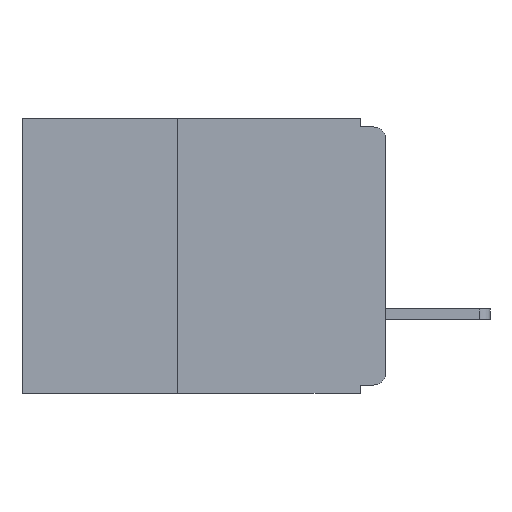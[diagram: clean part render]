
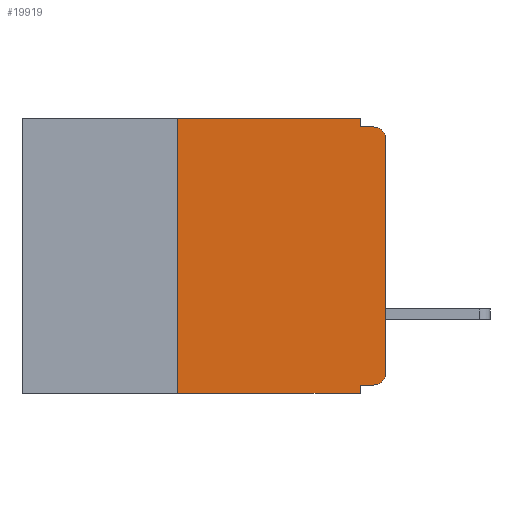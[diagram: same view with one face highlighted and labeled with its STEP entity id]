
A CAD part, left-side view. The second image highlights one B-rep face of the part: STEP entity #19919.
In plain terms, the highlighted planar face has unit normal (-1, 0, 0).
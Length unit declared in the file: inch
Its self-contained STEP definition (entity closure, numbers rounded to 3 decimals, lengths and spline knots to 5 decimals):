
#400 = LINE ( 'NONE', #5415, #15507 ) ;
#1231 = CARTESIAN_POINT ( 'NONE',  ( 0., 0., -0.305 ) ) ;
#1359 = EDGE_CURVE ( 'NONE', #19002, #3537, #1965, .T. ) ;
#1644 = CARTESIAN_POINT ( 'NONE',  ( 0., 0.031, -0.32 ) ) ;
#1772 = EDGE_CURVE ( 'NONE', #5327, #13326, #1940, .T. ) ;
#1792 = LINE ( 'NONE', #3826, #21398 ) ;
#1940 = LINE ( 'NONE', #8835, #17643 ) ;
#1965 = LINE ( 'NONE', #18386, #11450 ) ;
#2728 = ORIENTED_EDGE ( 'NONE', *, *, #5350, .F. ) ;
#2843 = CIRCLE ( 'NONE', #15401, 0.015 ) ;
#3136 = ORIENTED_EDGE ( 'NONE', *, *, #10812, .T. ) ;
#3235 = ORIENTED_EDGE ( 'NONE', *, *, #1772, .F. ) ;
#3537 = VERTEX_POINT ( 'NONE', #1644 ) ;
#3826 = CARTESIAN_POINT ( 'NONE',  ( 0., 0., 0. ) ) ;
#4131 = FACE_OUTER_BOUND ( 'NONE', #5495, .T. ) ;
#4585 = VECTOR ( 'NONE', #22225, 39.37008 ) ;
#4799 = CARTESIAN_POINT ( 'NONE',  ( 0., 0.25, -0.33 ) ) ;
#4830 = DIRECTION ( 'NONE',  ( -1., 0., 0. ) ) ;
#5327 = VERTEX_POINT ( 'NONE', #21970 ) ;
#5350 = EDGE_CURVE ( 'NONE', #16215, #5327, #21075, .T. ) ;
#5415 = CARTESIAN_POINT ( 'NONE',  ( 0., 0.437, -0.33 ) ) ;
#5495 = EDGE_LOOP ( 'NONE', ( #3136, #7941, #16570, #3235, #2728, #15216, #23591, #19054, #21875, #12855 ) ) ;
#5988 = CARTESIAN_POINT ( 'NONE',  ( 0., 0.25, 0. ) ) ;
#6038 = CARTESIAN_POINT ( 'NONE',  ( 0., 0.437, 0. ) ) ;
#7162 = VERTEX_POINT ( 'NONE', #1231 ) ;
#7653 = DIRECTION ( 'NONE',  ( 0., 0., 1. ) ) ;
#7763 = DIRECTION ( 'NONE',  ( 0., -1., 0. ) ) ;
#7941 = ORIENTED_EDGE ( 'NONE', *, *, #17765, .T. ) ;
#7986 = PLANE ( 'NONE',  #11604 ) ;
#8075 = DIRECTION ( 'NONE',  ( 0., 0., -1. ) ) ;
#8188 = CARTESIAN_POINT ( 'NONE',  ( 0., 0.015, -0.01 ) ) ;
#8351 = EDGE_CURVE ( 'NONE', #13326, #14379, #17920, .T. ) ;
#8835 = CARTESIAN_POINT ( 'NONE',  ( 0., 0.031, 0. ) ) ;
#8885 = DIRECTION ( 'NONE',  ( 0., 0., -1. ) ) ;
#9355 = VERTEX_POINT ( 'NONE', #14689 ) ;
#9783 = CARTESIAN_POINT ( 'NONE',  ( 0., 0.031, -0.33 ) ) ;
#10272 = LINE ( 'NONE', #12768, #4585 ) ;
#10615 = CIRCLE ( 'NONE', #12134, 0.015 ) ;
#10799 = VECTOR ( 'NONE', #23159, 39.37008 ) ;
#10812 = EDGE_CURVE ( 'NONE', #7162, #9355, #1792, .T. ) ;
#10923 = CARTESIAN_POINT ( 'NONE',  ( 0., 0.031, -0.01 ) ) ;
#11157 = DIRECTION ( 'NONE',  ( -1., 0., 0. ) ) ;
#11450 = VECTOR ( 'NONE', #18628, 39.37008 ) ;
#11604 = AXIS2_PLACEMENT_3D ( 'NONE', #6038, #19478, #8075 ) ;
#11620 = CARTESIAN_POINT ( 'NONE',  ( 0., 0., -0.01 ) ) ;
#11781 = EDGE_CURVE ( 'NONE', #19002, #7162, #10615, .T. ) ;
#12134 = AXIS2_PLACEMENT_3D ( 'NONE', #16259, #4830, #18157 ) ;
#12320 = VECTOR ( 'NONE', #7763, 39.37008 ) ;
#12443 = VERTEX_POINT ( 'NONE', #4799 ) ;
#12768 = CARTESIAN_POINT ( 'NONE',  ( 0., 0.25, -0.33 ) ) ;
#12855 = ORIENTED_EDGE ( 'NONE', *, *, #11781, .T. ) ;
#12989 = EDGE_CURVE ( 'NONE', #3537, #21159, #20930, .T. ) ;
#13326 = VERTEX_POINT ( 'NONE', #10923 ) ;
#14085 = EDGE_CURVE ( 'NONE', #12443, #21159, #400, .T. ) ;
#14379 = VERTEX_POINT ( 'NONE', #8188 ) ;
#14689 = CARTESIAN_POINT ( 'NONE',  ( 0., 0., -0.025 ) ) ;
#15216 = ORIENTED_EDGE ( 'NONE', *, *, #17654, .F. ) ;
#15401 = AXIS2_PLACEMENT_3D ( 'NONE', #22547, #11157, #24444 ) ;
#15507 = VECTOR ( 'NONE', #18767, 39.37008 ) ;
#15602 = CARTESIAN_POINT ( 'NONE',  ( 0., 0.031, -0.33 ) ) ;
#15998 = VECTOR ( 'NONE', #21528, 39.37008 ) ;
#16215 = VERTEX_POINT ( 'NONE', #5988 ) ;
#16259 = CARTESIAN_POINT ( 'NONE',  ( 0., 0.015, -0.305 ) ) ;
#16570 = ORIENTED_EDGE ( 'NONE', *, *, #8351, .F. ) ;
#17643 = VECTOR ( 'NONE', #8885, 39.37008 ) ;
#17654 = EDGE_CURVE ( 'NONE', #12443, #16215, #10272, .T. ) ;
#17765 = EDGE_CURVE ( 'NONE', #9355, #14379, #2843, .T. ) ;
#17920 = LINE ( 'NONE', #11620, #12320 ) ;
#18157 = DIRECTION ( 'NONE',  ( 0., 0., -1. ) ) ;
#18386 = CARTESIAN_POINT ( 'NONE',  ( 0., 0., -0.32 ) ) ;
#18628 = DIRECTION ( 'NONE',  ( 0., 1., 0. ) ) ;
#18767 = DIRECTION ( 'NONE',  ( 0., -1., 0. ) ) ;
#19002 = VERTEX_POINT ( 'NONE', #20197 ) ;
#19054 = ORIENTED_EDGE ( 'NONE', *, *, #12989, .F. ) ;
#19478 = DIRECTION ( 'NONE',  ( 1., 0., 0. ) ) ;
#19919 = ADVANCED_FACE ( 'NONE', ( #4131 ), #7986, .F. ) ;
#20197 = CARTESIAN_POINT ( 'NONE',  ( 0., 0.015, -0.32 ) ) ;
#20930 = LINE ( 'NONE', #15602, #10799 ) ;
#21075 = LINE ( 'NONE', #21583, #15998 ) ;
#21159 = VERTEX_POINT ( 'NONE', #9783 ) ;
#21398 = VECTOR ( 'NONE', #7653, 39.37008 ) ;
#21528 = DIRECTION ( 'NONE',  ( 0., -1., 0. ) ) ;
#21583 = CARTESIAN_POINT ( 'NONE',  ( 0., 0.437, 0. ) ) ;
#21875 = ORIENTED_EDGE ( 'NONE', *, *, #1359, .F. ) ;
#21970 = CARTESIAN_POINT ( 'NONE',  ( 0., 0.031, 0. ) ) ;
#22225 = DIRECTION ( 'NONE',  ( 0., 0., 1. ) ) ;
#22547 = CARTESIAN_POINT ( 'NONE',  ( 0., 0.015, -0.025 ) ) ;
#23159 = DIRECTION ( 'NONE',  ( 0., 0., -1. ) ) ;
#23591 = ORIENTED_EDGE ( 'NONE', *, *, #14085, .T. ) ;
#24444 = DIRECTION ( 'NONE',  ( 0., 0., -1. ) ) ;
